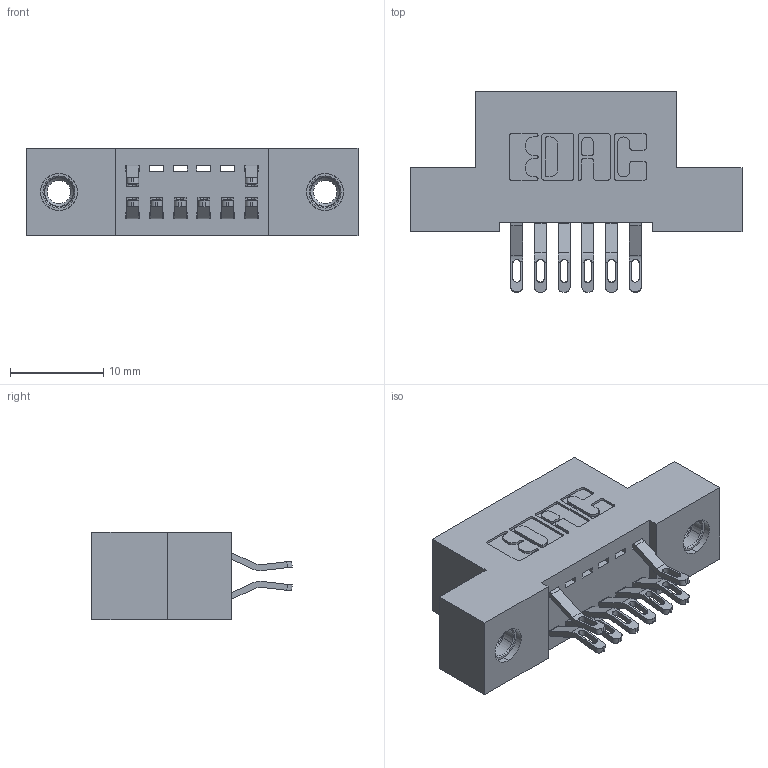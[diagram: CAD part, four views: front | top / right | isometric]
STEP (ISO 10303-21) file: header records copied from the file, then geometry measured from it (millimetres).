
FILE_DESCRIPTION (( 'STEP AP203' ), '1' );
FILE_NAME ('342-012-555-207.STEP', '2018-08-10T15:42:43', ( '' ), ( '' ), 'SwSTEP 2.0', 'SolidWorks 2016', '' );
FILE_SCHEMA (( 'CONFIG_CONTROL_DESIGN' ));
Length unit declared in the file: inch
Products named in the file (4): 342-012-555-207; 342 Part_TI; 345-292-001_555 Tail; 345-250-001_345-250-005-103
Assembly tree (11 placements, depth 2):
  342-012-555-207
    342 Part_TI
    345-292-001_555 Tail  x8
    345-250-001_345-250-005-103  x2
Bounding box: 35.56 x 21.47 x 9.4 mm (x, y, z)
Volume: 2998.2 mm3; surface area: 3897.5 mm2
Topology: 11 solids, 11 shells, 658 faces, 1983 edges, 1314 vertices
Faces by surface type: plane 394, cylinder 248, cone 12, torus 4
Entity records: 9768 total; most frequent: CARTESIAN_POINT 1695, ORIENTED_EDGE 1598, DIRECTION 1509, EDGE_CURVE 799, LINE 631, VECTOR 631, VERTEX_POINT 528, AXIS2_PLACEMENT_3D 439
